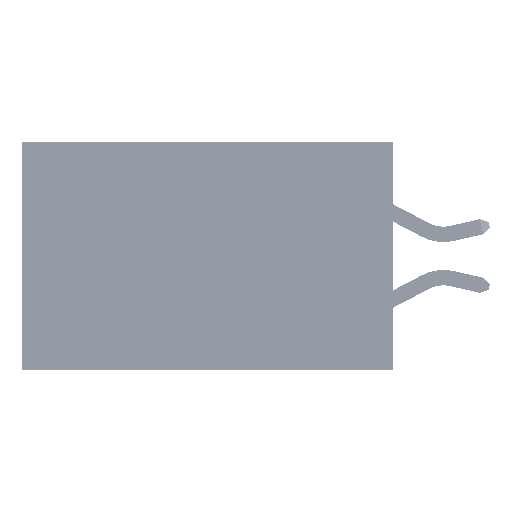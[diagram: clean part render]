
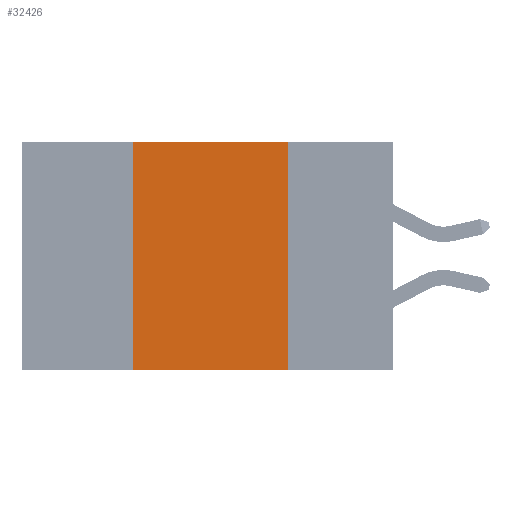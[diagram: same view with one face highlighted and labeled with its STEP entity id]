
A CAD part, left-side view. The second image highlights one B-rep face of the part: STEP entity #32426.
In plain terms, the highlighted planar face has unit normal (-1, 0, 0).
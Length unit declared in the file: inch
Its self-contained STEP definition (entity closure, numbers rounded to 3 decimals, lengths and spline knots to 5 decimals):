
#189 = VERTEX_POINT ( 'NONE', #22620 ) ;
#3996 = VECTOR ( 'NONE', #14403, 39.37008 ) ;
#5332 = CARTESIAN_POINT ( 'NONE',  ( 0., 0.6, -0.37 ) ) ;
#6056 = DIRECTION ( 'NONE',  ( 0., 0., -1. ) ) ;
#8077 = CARTESIAN_POINT ( 'NONE',  ( 0., 0.17, 0. ) ) ;
#9397 = CARTESIAN_POINT ( 'NONE',  ( 0., 0.6, 0. ) ) ;
#9603 = VECTOR ( 'NONE', #44590, 39.37008 ) ;
#11096 = VERTEX_POINT ( 'NONE', #8077 ) ;
#14403 = DIRECTION ( 'NONE',  ( 0., 0., 1. ) ) ;
#14439 = AXIS2_PLACEMENT_3D ( 'NONE', #9397, #41307, #16580 ) ;
#14613 = VECTOR ( 'NONE', #6056, 39.37008 ) ;
#16580 = DIRECTION ( 'NONE',  ( 0., 0., -1. ) ) ;
#17510 = FACE_OUTER_BOUND ( 'NONE', #42828, .T. ) ;
#18141 = EDGE_CURVE ( 'NONE', #189, #32924, #38148, .T. ) ;
#18311 = EDGE_CURVE ( 'NONE', #189, #21110, #20744, .T. ) ;
#19800 = ORIENTED_EDGE ( 'NONE', *, *, #18141, .T. ) ;
#20744 = LINE ( 'NONE', #41766, #3996 ) ;
#21110 = VERTEX_POINT ( 'NONE', #22819 ) ;
#22620 = CARTESIAN_POINT ( 'NONE',  ( 0., 0.42, -0.37 ) ) ;
#22819 = CARTESIAN_POINT ( 'NONE',  ( 0., 0.42, 0. ) ) ;
#23664 = DIRECTION ( 'NONE',  ( 0., -1., 0. ) ) ;
#24811 = LINE ( 'NONE', #41821, #36577 ) ;
#26228 = CARTESIAN_POINT ( 'NONE',  ( 0., 0.17, -0.37 ) ) ;
#30970 = PLANE ( 'NONE',  #14439 ) ;
#31758 = EDGE_CURVE ( 'NONE', #21110, #11096, #24811, .T. ) ;
#32426 = ADVANCED_FACE ( 'NONE', ( #17510 ), #30970, .F. ) ;
#32924 = VERTEX_POINT ( 'NONE', #26228 ) ;
#33146 = EDGE_CURVE ( 'NONE', #11096, #32924, #43697, .T. ) ;
#35566 = ORIENTED_EDGE ( 'NONE', *, *, #33146, .F. ) ;
#36577 = VECTOR ( 'NONE', #23664, 39.37008 ) ;
#37024 = ORIENTED_EDGE ( 'NONE', *, *, #31758, .F. ) ;
#38148 = LINE ( 'NONE', #5332, #9603 ) ;
#41307 = DIRECTION ( 'NONE',  ( 1., 0., 0. ) ) ;
#41721 = CARTESIAN_POINT ( 'NONE',  ( 0., 0.17, 0. ) ) ;
#41766 = CARTESIAN_POINT ( 'NONE',  ( 0., 0.42, 0. ) ) ;
#41821 = CARTESIAN_POINT ( 'NONE',  ( 0., 0.6, 0. ) ) ;
#42828 = EDGE_LOOP ( 'NONE', ( #35566, #37024, #43520, #19800 ) ) ;
#43520 = ORIENTED_EDGE ( 'NONE', *, *, #18311, .F. ) ;
#43697 = LINE ( 'NONE', #41721, #14613 ) ;
#44590 = DIRECTION ( 'NONE',  ( 0., -1., 0. ) ) ;
